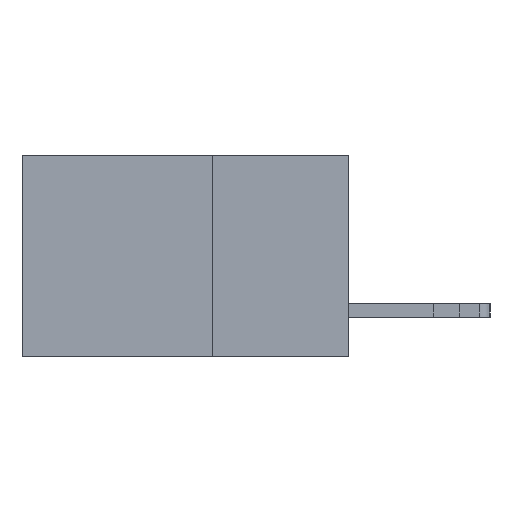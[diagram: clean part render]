
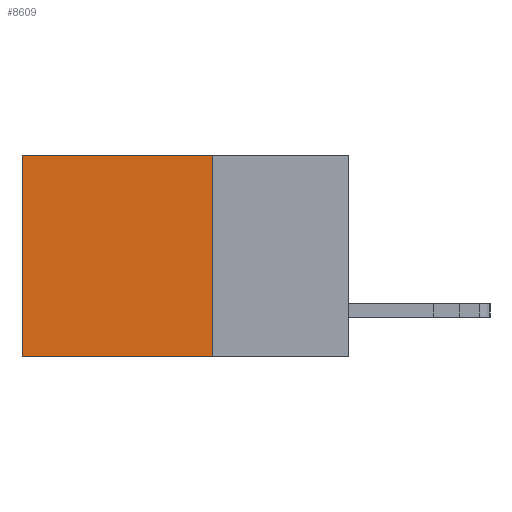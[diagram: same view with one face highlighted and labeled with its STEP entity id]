
A CAD part, left-side view. The second image highlights one B-rep face of the part: STEP entity #8609.
In plain terms, the highlighted planar face has unit normal (-1, 0, 0).
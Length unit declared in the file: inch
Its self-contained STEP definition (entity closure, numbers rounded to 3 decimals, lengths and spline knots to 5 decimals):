
#455 = CARTESIAN_POINT ( 'NONE',  ( 0.298, 0.6, -0.37 ) ) ;
#471 = ORIENTED_EDGE ( 'NONE', *, *, #14532, .F. ) ;
#957 = ORIENTED_EDGE ( 'NONE', *, *, #1838, .F. ) ;
#1016 = VECTOR ( 'NONE', #4955, 39.37008 ) ;
#1544 = LINE ( 'NONE', #1595, #15598 ) ;
#1595 = CARTESIAN_POINT ( 'NONE',  ( 0.298, 0.25, 0. ) ) ;
#1838 = EDGE_CURVE ( 'NONE', #4608, #8188, #1544, .T. ) ;
#2036 = EDGE_LOOP ( 'NONE', ( #2099, #471, #957, #9380 ) ) ;
#2099 = ORIENTED_EDGE ( 'NONE', *, *, #14375, .T. ) ;
#2144 = DIRECTION ( 'NONE',  ( 0., 0., -1. ) ) ;
#2750 = DIRECTION ( 'NONE',  ( 1., 0., 0. ) ) ;
#3365 = DIRECTION ( 'NONE',  ( 0., 1., 0. ) ) ;
#4608 = VERTEX_POINT ( 'NONE', #15232 ) ;
#4687 = LINE ( 'NONE', #10319, #1016 ) ;
#4699 = LINE ( 'NONE', #12853, #15526 ) ;
#4730 = VERTEX_POINT ( 'NONE', #8673 ) ;
#4955 = DIRECTION ( 'NONE',  ( 0., 1., 0. ) ) ;
#7362 = DIRECTION ( 'NONE',  ( 0., 0., -1. ) ) ;
#7626 = VECTOR ( 'NONE', #7362, 39.37008 ) ;
#8188 = VERTEX_POINT ( 'NONE', #9986 ) ;
#8609 = ADVANCED_FACE ( 'NONE', ( #10032 ), #14929, .F. ) ;
#8673 = CARTESIAN_POINT ( 'NONE',  ( 0.298, 0.6, 0. ) ) ;
#9380 = ORIENTED_EDGE ( 'NONE', *, *, #17371, .T. ) ;
#9986 = CARTESIAN_POINT ( 'NONE',  ( 0.298, 0.25, -0.37 ) ) ;
#10032 = FACE_OUTER_BOUND ( 'NONE', #2036, .T. ) ;
#10319 = CARTESIAN_POINT ( 'NONE',  ( 0.298, 0.25, -0.37 ) ) ;
#10336 = VERTEX_POINT ( 'NONE', #455 ) ;
#10859 = CARTESIAN_POINT ( 'NONE',  ( 0.298, 0.25, 0. ) ) ;
#12212 = DIRECTION ( 'NONE',  ( 0., 0., -1. ) ) ;
#12853 = CARTESIAN_POINT ( 'NONE',  ( 0.298, 0.25, 0. ) ) ;
#14018 = LINE ( 'NONE', #15517, #7626 ) ;
#14375 = EDGE_CURVE ( 'NONE', #4730, #10336, #14018, .T. ) ;
#14532 = EDGE_CURVE ( 'NONE', #8188, #10336, #4687, .T. ) ;
#14564 = AXIS2_PLACEMENT_3D ( 'NONE', #10859, #2750, #12212 ) ;
#14929 = PLANE ( 'NONE',  #14564 ) ;
#15232 = CARTESIAN_POINT ( 'NONE',  ( 0.298, 0.25, 0. ) ) ;
#15517 = CARTESIAN_POINT ( 'NONE',  ( 0.298, 0.6, 0. ) ) ;
#15526 = VECTOR ( 'NONE', #3365, 39.37008 ) ;
#15598 = VECTOR ( 'NONE', #2144, 39.37008 ) ;
#17371 = EDGE_CURVE ( 'NONE', #4608, #4730, #4699, .T. ) ;
